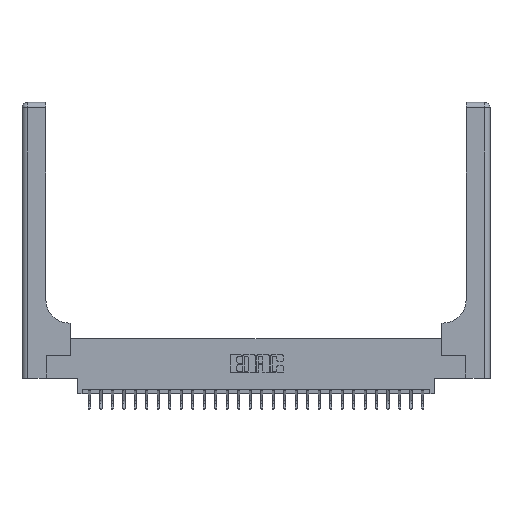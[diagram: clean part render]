
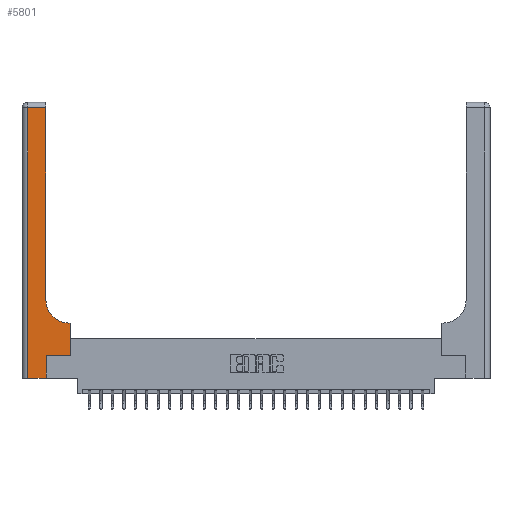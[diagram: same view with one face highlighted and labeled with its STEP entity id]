
A CAD part, top view. The second image highlights one B-rep face of the part: STEP entity #5801.
In plain terms, the highlighted planar face has unit normal (0, 0, 1).
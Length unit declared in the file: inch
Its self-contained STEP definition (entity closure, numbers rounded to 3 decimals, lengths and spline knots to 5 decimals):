
#479 = DIRECTION ( 'NONE',  ( 0., -1., 0. ) ) ;
#788 = LINE ( 'NONE', #6960, #9459 ) ;
#855 = FACE_OUTER_BOUND ( 'NONE', #11209, .T. ) ;
#1315 = EDGE_CURVE ( 'NONE', #3858, #20495, #18517, .T. ) ;
#1431 = CARTESIAN_POINT ( 'NONE',  ( 0.06, 0., 0.37 ) ) ;
#2126 = ORIENTED_EDGE ( 'NONE', *, *, #16937, .T. ) ;
#2652 = DIRECTION ( 'NONE',  ( 0., 1., 0. ) ) ;
#2658 = VECTOR ( 'NONE', #22879, 39.37008 ) ;
#2708 = ORIENTED_EDGE ( 'NONE', *, *, #5192, .T. ) ;
#2773 = LINE ( 'NONE', #6888, #15253 ) ;
#3453 = LINE ( 'NONE', #18184, #9690 ) ;
#3781 = DIRECTION ( 'NONE',  ( 0., 1., 0. ) ) ;
#3858 = VERTEX_POINT ( 'NONE', #11751 ) ;
#4826 = PLANE ( 'NONE',  #16317 ) ;
#5100 = DIRECTION ( 'NONE',  ( -1., 0., 0. ) ) ;
#5192 = EDGE_CURVE ( 'NONE', #13938, #16472, #17555, .T. ) ;
#5248 = VECTOR ( 'NONE', #20753, 39.37008 ) ;
#5801 = ADVANCED_FACE ( 'NONE', ( #855 ), #4826, .F. ) ;
#5985 = CARTESIAN_POINT ( 'NONE',  ( 0.51, 0.6, 0.37 ) ) ;
#6483 = CIRCLE ( 'NONE', #20600, 0.25 ) ;
#6888 = CARTESIAN_POINT ( 'NONE',  ( 0.26, 3., 0.37 ) ) ;
#6950 = CARTESIAN_POINT ( 'NONE',  ( 0.26, 0.85, 0.37 ) ) ;
#6960 = CARTESIAN_POINT ( 'NONE',  ( 0.528, 0.25, 0.37 ) ) ;
#7590 = DIRECTION ( 'NONE',  ( -1., 0., 0. ) ) ;
#7591 = ORIENTED_EDGE ( 'NONE', *, *, #16549, .T. ) ;
#8077 = CARTESIAN_POINT ( 'NONE',  ( 0.265, 0.25, 0.37 ) ) ;
#9350 = ORIENTED_EDGE ( 'NONE', *, *, #1315, .T. ) ;
#9459 = VECTOR ( 'NONE', #25583, 39.37008 ) ;
#9554 = VECTOR ( 'NONE', #479, 39.37008 ) ;
#9690 = VECTOR ( 'NONE', #20009, 39.37008 ) ;
#10561 = ORIENTED_EDGE ( 'NONE', *, *, #15026, .T. ) ;
#11209 = EDGE_LOOP ( 'NONE', ( #12580, #7591, #2708, #10561, #9350, #16137, #22682, #2126, #14330 ) ) ;
#11746 = CARTESIAN_POINT ( 'NONE',  ( 0., 2.94, 0.37 ) ) ;
#11751 = CARTESIAN_POINT ( 'NONE',  ( 0.265, 0., 0.37 ) ) ;
#12261 = VECTOR ( 'NONE', #3781, 39.37008 ) ;
#12580 = ORIENTED_EDGE ( 'NONE', *, *, #24646, .T. ) ;
#13249 = EDGE_CURVE ( 'NONE', #20495, #20518, #24660, .T. ) ;
#13901 = VERTEX_POINT ( 'NONE', #6950 ) ;
#13938 = VERTEX_POINT ( 'NONE', #15638 ) ;
#14120 = LINE ( 'NONE', #16051, #5248 ) ;
#14222 = CARTESIAN_POINT ( 'NONE',  ( 0.26, 2.94, 0.37 ) ) ;
#14330 = ORIENTED_EDGE ( 'NONE', *, *, #17986, .T. ) ;
#15026 = EDGE_CURVE ( 'NONE', #16472, #3858, #14120, .T. ) ;
#15253 = VECTOR ( 'NONE', #2652, 39.37008 ) ;
#15591 = DIRECTION ( 'NONE',  ( 1., 0., 0. ) ) ;
#15638 = CARTESIAN_POINT ( 'NONE',  ( 0.06, 2.94, 0.37 ) ) ;
#15871 = DIRECTION ( 'NONE',  ( 0., 0., -1. ) ) ;
#16051 = CARTESIAN_POINT ( 'NONE',  ( 0., 0., 0.37 ) ) ;
#16137 = ORIENTED_EDGE ( 'NONE', *, *, #13249, .T. ) ;
#16317 = AXIS2_PLACEMENT_3D ( 'NONE', #23887, #26208, #5100 ) ;
#16472 = VERTEX_POINT ( 'NONE', #1431 ) ;
#16549 = EDGE_CURVE ( 'NONE', #25758, #13938, #18359, .T. ) ;
#16600 = VERTEX_POINT ( 'NONE', #20595 ) ;
#16690 = CARTESIAN_POINT ( 'NONE',  ( 0.528, 0.25, 0.37 ) ) ;
#16937 = EDGE_CURVE ( 'NONE', #16600, #21371, #3453, .T. ) ;
#17555 = LINE ( 'NONE', #21855, #9554 ) ;
#17986 = EDGE_CURVE ( 'NONE', #21371, #13901, #6483, .T. ) ;
#18184 = CARTESIAN_POINT ( 'NONE',  ( 0.26, 0.6, 0.37 ) ) ;
#18359 = LINE ( 'NONE', #11746, #26558 ) ;
#18517 = LINE ( 'NONE', #22540, #12261 ) ;
#20009 = DIRECTION ( 'NONE',  ( -1., 0., 0. ) ) ;
#20495 = VERTEX_POINT ( 'NONE', #25215 ) ;
#20518 = VERTEX_POINT ( 'NONE', #16690 ) ;
#20595 = CARTESIAN_POINT ( 'NONE',  ( 0.528, 0.6, 0.37 ) ) ;
#20600 = AXIS2_PLACEMENT_3D ( 'NONE', #26073, #15871, #15591 ) ;
#20753 = DIRECTION ( 'NONE',  ( 1., 0., 0. ) ) ;
#21371 = VERTEX_POINT ( 'NONE', #5985 ) ;
#21855 = CARTESIAN_POINT ( 'NONE',  ( 0.06, 3., 0.37 ) ) ;
#22540 = CARTESIAN_POINT ( 'NONE',  ( 0.265, 0., 0.37 ) ) ;
#22682 = ORIENTED_EDGE ( 'NONE', *, *, #26959, .T. ) ;
#22879 = DIRECTION ( 'NONE',  ( 1., 0., 0. ) ) ;
#23887 = CARTESIAN_POINT ( 'NONE',  ( 0., 3., 0.37 ) ) ;
#24646 = EDGE_CURVE ( 'NONE', #13901, #25758, #2773, .T. ) ;
#24660 = LINE ( 'NONE', #8077, #2658 ) ;
#25215 = CARTESIAN_POINT ( 'NONE',  ( 0.265, 0.25, 0.37 ) ) ;
#25583 = DIRECTION ( 'NONE',  ( 0., 1., 0. ) ) ;
#25758 = VERTEX_POINT ( 'NONE', #14222 ) ;
#26073 = CARTESIAN_POINT ( 'NONE',  ( 0.51, 0.85, 0.37 ) ) ;
#26208 = DIRECTION ( 'NONE',  ( 0., 0., -1. ) ) ;
#26558 = VECTOR ( 'NONE', #7590, 39.37008 ) ;
#26959 = EDGE_CURVE ( 'NONE', #20518, #16600, #788, .T. ) ;
